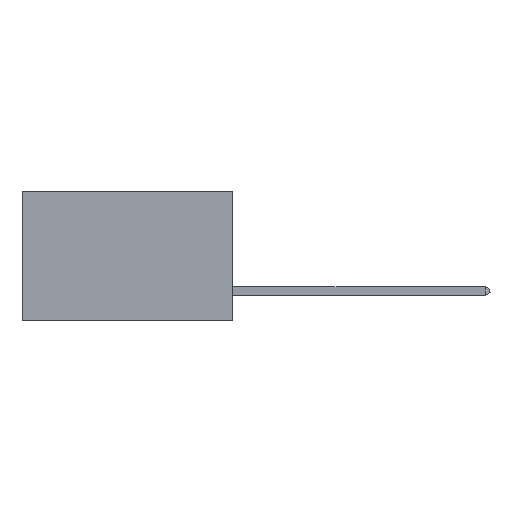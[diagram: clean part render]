
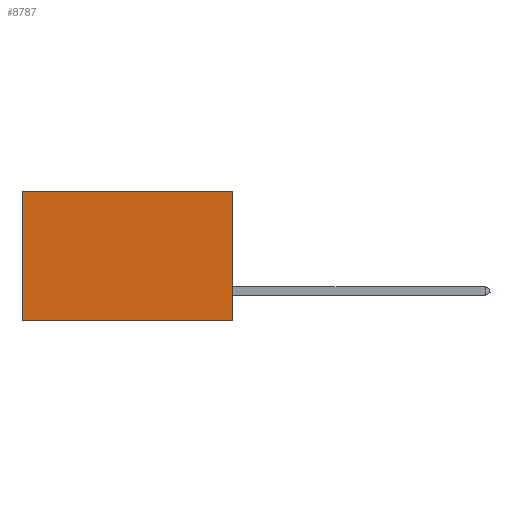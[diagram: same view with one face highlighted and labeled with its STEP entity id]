
A CAD part, left-side view. The second image highlights one B-rep face of the part: STEP entity #8787.
In plain terms, the highlighted planar face has unit normal (-1, 0, 0).
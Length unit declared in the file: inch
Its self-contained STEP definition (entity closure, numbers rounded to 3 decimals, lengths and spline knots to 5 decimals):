
#1216 = LINE ( 'NONE', #27643, #2890 ) ;
#1568 = VECTOR ( 'NONE', #43441, 39.37008 ) ;
#1711 = EDGE_CURVE ( 'NONE', #30035, #32115, #7565, .T. ) ;
#2845 = ORIENTED_EDGE ( 'NONE', *, *, #1711, .F. ) ;
#2890 = VECTOR ( 'NONE', #5693, 39.37008 ) ;
#3769 = VERTEX_POINT ( 'NONE', #18000 ) ;
#4688 = VECTOR ( 'NONE', #43040, 39.37008 ) ;
#5693 = DIRECTION ( 'NONE',  ( 0., 0., -1. ) ) ;
#7448 = CARTESIAN_POINT ( 'NONE',  ( 0.2875, 0.6, -0.37 ) ) ;
#7565 = LINE ( 'NONE', #30736, #18437 ) ;
#7951 = ORIENTED_EDGE ( 'NONE', *, *, #23202, .T. ) ;
#8787 = ADVANCED_FACE ( 'NONE', ( #23473 ), #28076, .F. ) ;
#10353 = CARTESIAN_POINT ( 'NONE',  ( 0.2875, 0., 0. ) ) ;
#14068 = VERTEX_POINT ( 'NONE', #28303 ) ;
#15546 = LINE ( 'NONE', #39688, #4688 ) ;
#17025 = DIRECTION ( 'NONE',  ( 0., 0., -1. ) ) ;
#18000 = CARTESIAN_POINT ( 'NONE',  ( 0.2875, 0., 0. ) ) ;
#18437 = VECTOR ( 'NONE', #27487, 39.37008 ) ;
#23202 = EDGE_CURVE ( 'NONE', #3769, #14068, #43283, .T. ) ;
#23473 = FACE_OUTER_BOUND ( 'NONE', #38738, .T. ) ;
#24215 = ORIENTED_EDGE ( 'NONE', *, *, #43087, .F. ) ;
#24847 = DIRECTION ( 'NONE',  ( 1., 0., 0. ) ) ;
#25281 = CARTESIAN_POINT ( 'NONE',  ( 0.2875, 0., -0.37 ) ) ;
#27487 = DIRECTION ( 'NONE',  ( 0., 1., 0. ) ) ;
#27643 = CARTESIAN_POINT ( 'NONE',  ( 0.2875, 0., 0. ) ) ;
#28076 = PLANE ( 'NONE',  #46398 ) ;
#28303 = CARTESIAN_POINT ( 'NONE',  ( 0.2875, 0.6, 0. ) ) ;
#28384 = CARTESIAN_POINT ( 'NONE',  ( 0.2875, 0., 0. ) ) ;
#30035 = VERTEX_POINT ( 'NONE', #25281 ) ;
#30736 = CARTESIAN_POINT ( 'NONE',  ( 0.2875, 0., -0.37 ) ) ;
#30804 = EDGE_CURVE ( 'NONE', #14068, #32115, #15546, .T. ) ;
#32115 = VERTEX_POINT ( 'NONE', #7448 ) ;
#38738 = EDGE_LOOP ( 'NONE', ( #39502, #2845, #24215, #7951 ) ) ;
#39502 = ORIENTED_EDGE ( 'NONE', *, *, #30804, .T. ) ;
#39688 = CARTESIAN_POINT ( 'NONE',  ( 0.2875, 0.6, 0. ) ) ;
#43040 = DIRECTION ( 'NONE',  ( 0., 0., -1. ) ) ;
#43087 = EDGE_CURVE ( 'NONE', #3769, #30035, #1216, .T. ) ;
#43283 = LINE ( 'NONE', #10353, #1568 ) ;
#43441 = DIRECTION ( 'NONE',  ( 0., 1., 0. ) ) ;
#46398 = AXIS2_PLACEMENT_3D ( 'NONE', #28384, #24847, #17025 ) ;
